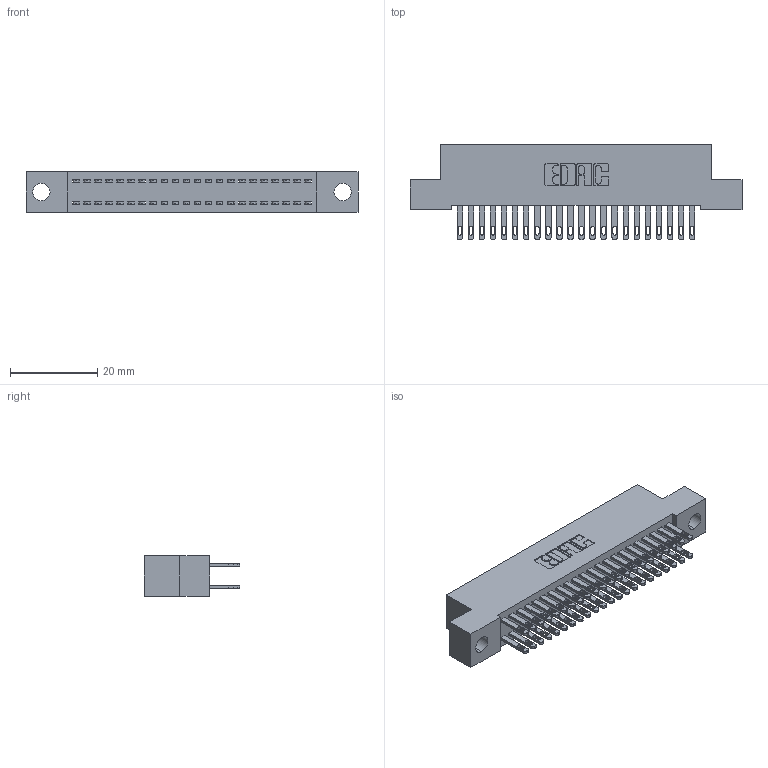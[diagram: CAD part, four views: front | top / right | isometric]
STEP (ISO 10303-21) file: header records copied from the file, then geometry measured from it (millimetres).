
FILE_DESCRIPTION (( 'STEP AP203' ), '1' );
FILE_NAME ('892-044-500-204.STEP', '2020-09-21T17:01:37', ( '' ), ( '' ), 'SwSTEP 2.0', 'SolidWorks 2020', '' );
FILE_SCHEMA (( 'CONFIG_CONTROL_DESIGN' ));
Length unit declared in the file: inch
Products named in the file (3): 892-044-500-204; 842 Part_.156 TH; 345-292-001_345-293-100
Assembly tree (45 placements, depth 2):
  892-044-500-204
    842 Part_.156 TH
    345-292-001_345-293-100  x44
Bounding box: 76.2 x 21.85 x 9.4 mm (x, y, z)
Volume: 6799.3 mm3; surface area: 10820.3 mm2
Topology: 45 solids, 45 shells, 2222 faces, 6767 edges, 4510 vertices
Faces by surface type: plane 1386, cylinder 836
Entity records: 16541 total; most frequent: CARTESIAN_POINT 2762, ORIENTED_EDGE 2698, DIRECTION 2397, EDGE_CURVE 1349, VECTOR 1217, LINE 1217, VERTEX_POINT 898, AXIS2_PLACEMENT_3D 590
